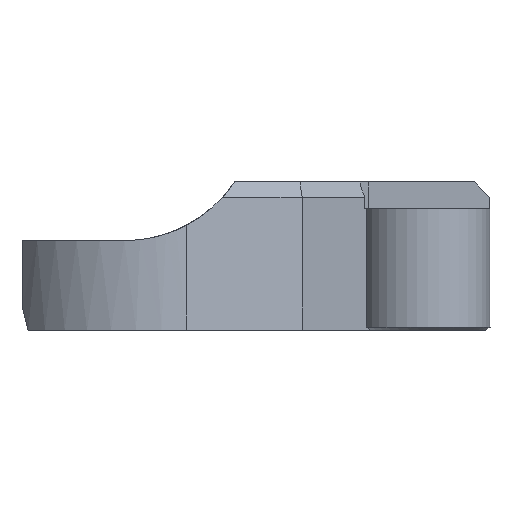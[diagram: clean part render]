
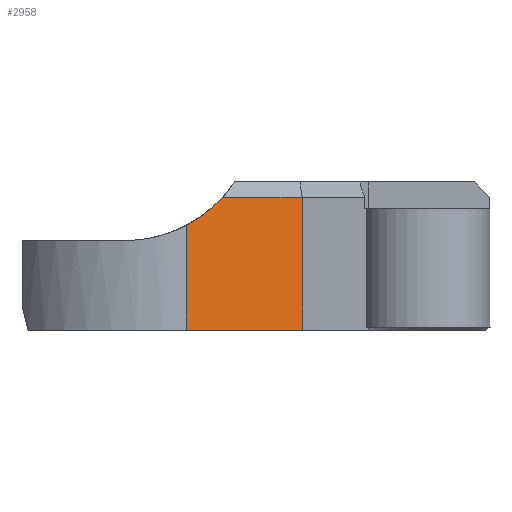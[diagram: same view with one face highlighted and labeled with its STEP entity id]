
A CAD part, front view. The second image highlights one B-rep face of the part: STEP entity #2958.
In plain terms, the highlighted planar face has unit normal (0.279, -0.96, 0).
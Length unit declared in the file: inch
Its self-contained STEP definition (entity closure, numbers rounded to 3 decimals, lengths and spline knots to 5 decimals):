
#44 = VERTEX_POINT ( 'NONE', #8164 ) ;
#186 = CARTESIAN_POINT ( 'NONE',  ( 2.95141, -0.41071, 3.8892 ) ) ;
#362 = VERTEX_POINT ( 'NONE', #8370 ) ;
#372 = VERTEX_POINT ( 'NONE', #2314 ) ;
#437 = VECTOR ( 'NONE', #7420, 39.37008 ) ;
#705 = EDGE_CURVE ( 'NONE', #362, #372, #2994, .T. ) ;
#1160 = DIRECTION ( 'NONE',  ( 0., 0., -1. ) ) ;
#1268 = VECTOR ( 'NONE', #1160, 39.37008 ) ;
#1330 = DIRECTION ( 'NONE',  ( 0., 0., -1. ) ) ;
#1368 = DIRECTION ( 'NONE',  ( 0.279, -0.96, 0. ) ) ;
#1374 = EDGE_CURVE ( 'NONE', #362, #7170, #8376, .T. ) ;
#1510 = CARTESIAN_POINT ( 'NONE',  ( 3.07817, -0.37391, 4.00548 ) ) ;
#1908 = LINE ( 'NONE', #4331, #2671 ) ;
#1916 = CARTESIAN_POINT ( 'NONE',  ( 2.87502, -0.43289, 3.84899 ) ) ;
#2288 = EDGE_LOOP ( 'NONE', ( #6131, #8539, #8653, #7447, #2628 ) ) ;
#2314 = CARTESIAN_POINT ( 'NONE',  ( 3.07817, -0.37391, 4.00548 ) ) ;
#2628 = ORIENTED_EDGE ( 'NONE', *, *, #2972, .F. ) ;
#2671 = VECTOR ( 'NONE', #7710, 39.37008 ) ;
#2958 = ADVANCED_FACE ( 'NONE', ( #8262 ), #6941, .T. ) ;
#2972 = EDGE_CURVE ( 'NONE', #8481, #7170, #1908, .T. ) ;
#2994 =( BOUNDED_CURVE ( )  B_SPLINE_CURVE ( 3, ( #1916, #186, #3520, #1510 ),
 .UNSPECIFIED., .F., .T. ) 
 B_SPLINE_CURVE_WITH_KNOTS ( ( 4, 4 ),
 ( 5.19698, 5.54056 ),
 .UNSPECIFIED. ) 
 CURVE ( )  GEOMETRIC_REPRESENTATION_ITEM ( )  RATIONAL_B_SPLINE_CURVE ( ( 1., 0.99, 0.99, 1. ) ) 
 REPRESENTATION_ITEM ( '' )  );
#3228 = AXIS2_PLACEMENT_3D ( 'NONE', #7489, #1368, #6119 ) ;
#3498 = EDGE_CURVE ( 'NONE', #44, #372, #7433, .T. ) ;
#3520 = CARTESIAN_POINT ( 'NONE',  ( 3.01979, -0.39086, 3.94188 ) ) ;
#3982 = CARTESIAN_POINT ( 'NONE',  ( 3.52564, -0.24399, 6.36544 ) ) ;
#4331 = CARTESIAN_POINT ( 'NONE',  ( 3.52564, -0.24399, 3.25964 ) ) ;
#4879 = EDGE_CURVE ( 'NONE', #44, #8481, #6784, .T. ) ;
#5338 = CARTESIAN_POINT ( 'NONE',  ( 3.52564, -0.24399, 3.25964 ) ) ;
#6119 = DIRECTION ( 'NONE',  ( -0.96, -0.279, 0. ) ) ;
#6131 = ORIENTED_EDGE ( 'NONE', *, *, #4879, .F. ) ;
#6495 = VECTOR ( 'NONE', #1330, 39.37008 ) ;
#6784 = LINE ( 'NONE', #3982, #1268 ) ;
#6795 = CARTESIAN_POINT ( 'NONE',  ( 3.14724, -0.35385, 4.00548 ) ) ;
#6941 = PLANE ( 'NONE',  #3228 ) ;
#7170 = VERTEX_POINT ( 'NONE', #7247 ) ;
#7247 = CARTESIAN_POINT ( 'NONE',  ( 2.87502, -0.43289, 3.25964 ) ) ;
#7420 = DIRECTION ( 'NONE',  ( -0.96, -0.279, 0. ) ) ;
#7433 = LINE ( 'NONE', #6795, #437 ) ;
#7447 = ORIENTED_EDGE ( 'NONE', *, *, #1374, .T. ) ;
#7489 = CARTESIAN_POINT ( 'NONE',  ( 3.52564, -0.24399, 6.36544 ) ) ;
#7710 = DIRECTION ( 'NONE',  ( -0.96, -0.279, 0. ) ) ;
#8007 = CARTESIAN_POINT ( 'NONE',  ( 2.87502, -0.43289, 6.36544 ) ) ;
#8164 = CARTESIAN_POINT ( 'NONE',  ( 3.52564, -0.24399, 4.00548 ) ) ;
#8262 = FACE_OUTER_BOUND ( 'NONE', #2288, .T. ) ;
#8370 = CARTESIAN_POINT ( 'NONE',  ( 2.87502, -0.43289, 3.84899 ) ) ;
#8376 = LINE ( 'NONE', #8007, #6495 ) ;
#8481 = VERTEX_POINT ( 'NONE', #5338 ) ;
#8539 = ORIENTED_EDGE ( 'NONE', *, *, #3498, .T. ) ;
#8653 = ORIENTED_EDGE ( 'NONE', *, *, #705, .F. ) ;
